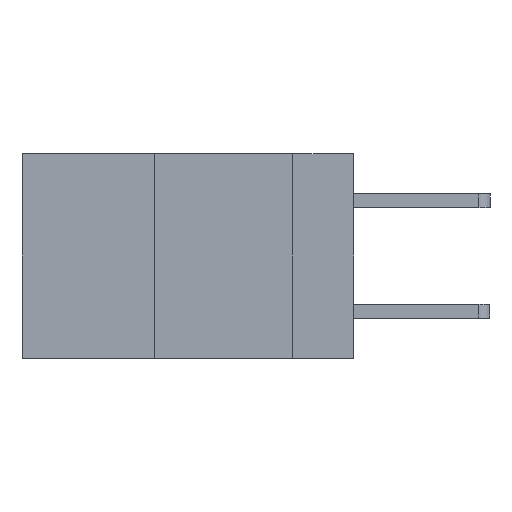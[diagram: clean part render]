
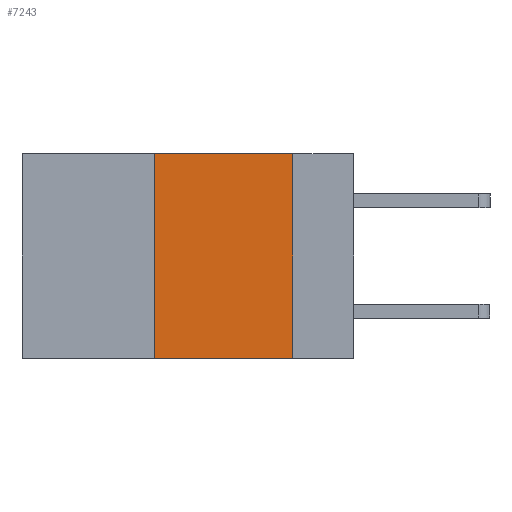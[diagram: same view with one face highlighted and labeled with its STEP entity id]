
A CAD part, left-side view. The second image highlights one B-rep face of the part: STEP entity #7243.
In plain terms, the highlighted planar face has unit normal (-1, 0, 0).
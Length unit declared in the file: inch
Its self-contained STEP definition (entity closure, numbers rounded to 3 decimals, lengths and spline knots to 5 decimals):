
#263 = CARTESIAN_POINT ( 'NONE',  ( 0., 0.6, 0. ) ) ;
#336 = ORIENTED_EDGE ( 'NONE', *, *, #6698, .T. ) ;
#919 = DIRECTION ( 'NONE',  ( 0., -1., 0. ) ) ;
#1159 = ORIENTED_EDGE ( 'NONE', *, *, #10725, .F. ) ;
#1237 = FACE_OUTER_BOUND ( 'NONE', #7892, .T. ) ;
#1513 = DIRECTION ( 'NONE',  ( 0., 0., -1. ) ) ;
#3093 = DIRECTION ( 'NONE',  ( 0., -1., 0. ) ) ;
#3141 = VECTOR ( 'NONE', #3093, 39.37008 ) ;
#3353 = DIRECTION ( 'NONE',  ( 0., 0., -1. ) ) ;
#3743 = EDGE_CURVE ( 'NONE', #6845, #9004, #10551, .T. ) ;
#5067 = CARTESIAN_POINT ( 'NONE',  ( 0., 0.11, -0.37 ) ) ;
#5243 = PLANE ( 'NONE',  #8763 ) ;
#5911 = LINE ( 'NONE', #10833, #3141 ) ;
#6041 = LINE ( 'NONE', #11340, #9848 ) ;
#6287 = VERTEX_POINT ( 'NONE', #7341 ) ;
#6289 = CARTESIAN_POINT ( 'NONE',  ( 0., 0.36, 0. ) ) ;
#6698 = EDGE_CURVE ( 'NONE', #6287, #12518, #5911, .T. ) ;
#6845 = VERTEX_POINT ( 'NONE', #6289 ) ;
#7243 = ADVANCED_FACE ( 'NONE', ( #1237 ), #5243, .F. ) ;
#7341 = CARTESIAN_POINT ( 'NONE',  ( 0., 0.36, -0.37 ) ) ;
#7580 = LINE ( 'NONE', #12232, #9678 ) ;
#7892 = EDGE_LOOP ( 'NONE', ( #1159, #9376, #8309, #336 ) ) ;
#8152 = DIRECTION ( 'NONE',  ( 1., 0., 0. ) ) ;
#8196 = CARTESIAN_POINT ( 'NONE',  ( 0., 0.11, 0. ) ) ;
#8309 = ORIENTED_EDGE ( 'NONE', *, *, #12672, .F. ) ;
#8364 = DIRECTION ( 'NONE',  ( 0., 0., 1. ) ) ;
#8763 = AXIS2_PLACEMENT_3D ( 'NONE', #263, #8152, #3353 ) ;
#9004 = VERTEX_POINT ( 'NONE', #8196 ) ;
#9376 = ORIENTED_EDGE ( 'NONE', *, *, #3743, .F. ) ;
#9678 = VECTOR ( 'NONE', #8364, 39.37008 ) ;
#9848 = VECTOR ( 'NONE', #1513, 39.37008 ) ;
#10377 = VECTOR ( 'NONE', #919, 39.37008 ) ;
#10551 = LINE ( 'NONE', #11717, #10377 ) ;
#10725 = EDGE_CURVE ( 'NONE', #9004, #12518, #6041, .T. ) ;
#10833 = CARTESIAN_POINT ( 'NONE',  ( 0., 0.6, -0.37 ) ) ;
#11340 = CARTESIAN_POINT ( 'NONE',  ( 0., 0.11, 0. ) ) ;
#11717 = CARTESIAN_POINT ( 'NONE',  ( 0., 0.6, 0. ) ) ;
#12232 = CARTESIAN_POINT ( 'NONE',  ( 0., 0.36, 0. ) ) ;
#12518 = VERTEX_POINT ( 'NONE', #5067 ) ;
#12672 = EDGE_CURVE ( 'NONE', #6287, #6845, #7580, .T. ) ;
